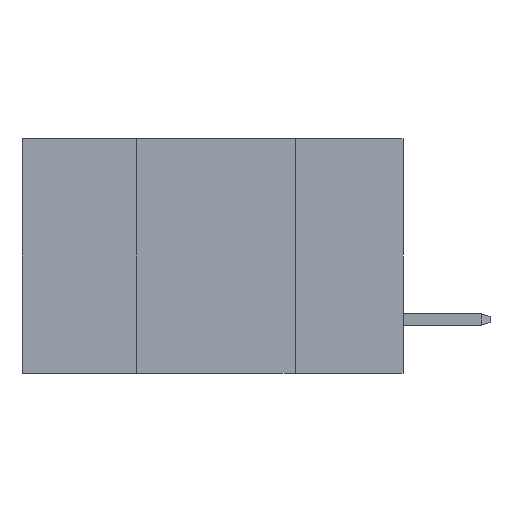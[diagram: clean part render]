
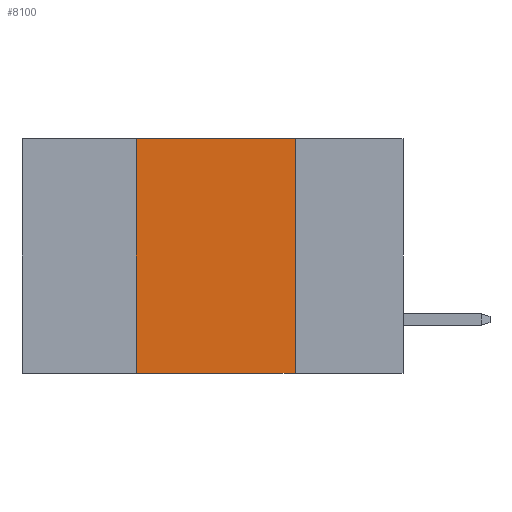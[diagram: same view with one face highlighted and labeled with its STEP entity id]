
A CAD part, left-side view. The second image highlights one B-rep face of the part: STEP entity #8100.
In plain terms, the highlighted planar face has unit normal (-1, 0, 0).
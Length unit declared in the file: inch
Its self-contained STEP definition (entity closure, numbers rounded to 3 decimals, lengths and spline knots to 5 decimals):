
#197 = FACE_OUTER_BOUND ( 'NONE', #9675, .T. ) ;
#814 = DIRECTION ( 'NONE',  ( 0., -1., 0. ) ) ;
#934 = EDGE_CURVE ( 'NONE', #1460, #9770, #7172, .T. ) ;
#1126 = PLANE ( 'NONE',  #8105 ) ;
#1410 = DIRECTION ( 'NONE',  ( 0., 0., -1. ) ) ;
#1460 = VERTEX_POINT ( 'NONE', #3828 ) ;
#1886 = CARTESIAN_POINT ( 'NONE',  ( 0., 0.42, 0. ) ) ;
#2109 = ORIENTED_EDGE ( 'NONE', *, *, #8852, .F. ) ;
#2688 = VECTOR ( 'NONE', #3109, 39.37008 ) ;
#2949 = CARTESIAN_POINT ( 'NONE',  ( 0., 0.6, 0. ) ) ;
#3064 = EDGE_CURVE ( 'NONE', #7510, #9770, #8289, .T. ) ;
#3109 = DIRECTION ( 'NONE',  ( 0., -1., 0. ) ) ;
#3267 = ORIENTED_EDGE ( 'NONE', *, *, #934, .T. ) ;
#3281 = CARTESIAN_POINT ( 'NONE',  ( 0., 0.6, -0.37 ) ) ;
#3282 = VECTOR ( 'NONE', #814, 39.37008 ) ;
#3524 = CARTESIAN_POINT ( 'NONE',  ( 0., 0.17, 0. ) ) ;
#3777 = EDGE_CURVE ( 'NONE', #1460, #6068, #7145, .T. ) ;
#3828 = CARTESIAN_POINT ( 'NONE',  ( 0., 0.42, -0.37 ) ) ;
#4426 = CARTESIAN_POINT ( 'NONE',  ( 0., 0.17, 0. ) ) ;
#4631 = ORIENTED_EDGE ( 'NONE', *, *, #3064, .F. ) ;
#4663 = VECTOR ( 'NONE', #7981, 39.37008 ) ;
#4841 = VECTOR ( 'NONE', #1410, 39.37008 ) ;
#4858 = CARTESIAN_POINT ( 'NONE',  ( 0., 0.17, -0.37 ) ) ;
#4916 = DIRECTION ( 'NONE',  ( 0., 0., -1. ) ) ;
#6068 = VERTEX_POINT ( 'NONE', #1886 ) ;
#7145 = LINE ( 'NONE', #8893, #4663 ) ;
#7172 = LINE ( 'NONE', #3281, #3282 ) ;
#7279 = DIRECTION ( 'NONE',  ( 1., 0., 0. ) ) ;
#7510 = VERTEX_POINT ( 'NONE', #3524 ) ;
#7981 = DIRECTION ( 'NONE',  ( 0., 0., 1. ) ) ;
#8100 = ADVANCED_FACE ( 'NONE', ( #197 ), #1126, .F. ) ;
#8105 = AXIS2_PLACEMENT_3D ( 'NONE', #9603, #7279, #4916 ) ;
#8289 = LINE ( 'NONE', #4426, #4841 ) ;
#8558 = ORIENTED_EDGE ( 'NONE', *, *, #3777, .F. ) ;
#8852 = EDGE_CURVE ( 'NONE', #6068, #7510, #9367, .T. ) ;
#8893 = CARTESIAN_POINT ( 'NONE',  ( 0., 0.42, 0. ) ) ;
#9367 = LINE ( 'NONE', #2949, #2688 ) ;
#9603 = CARTESIAN_POINT ( 'NONE',  ( 0., 0.6, 0. ) ) ;
#9675 = EDGE_LOOP ( 'NONE', ( #4631, #2109, #8558, #3267 ) ) ;
#9770 = VERTEX_POINT ( 'NONE', #4858 ) ;
